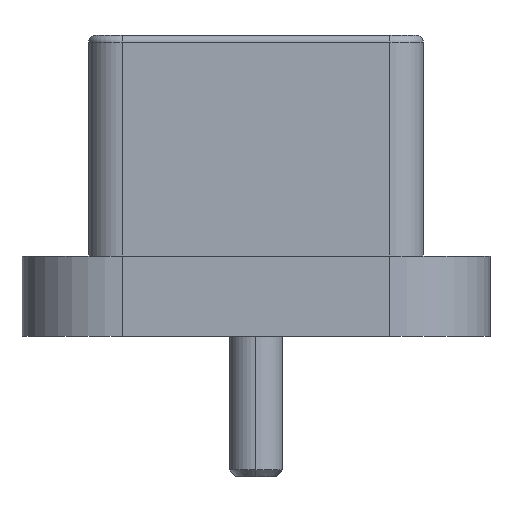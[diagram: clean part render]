
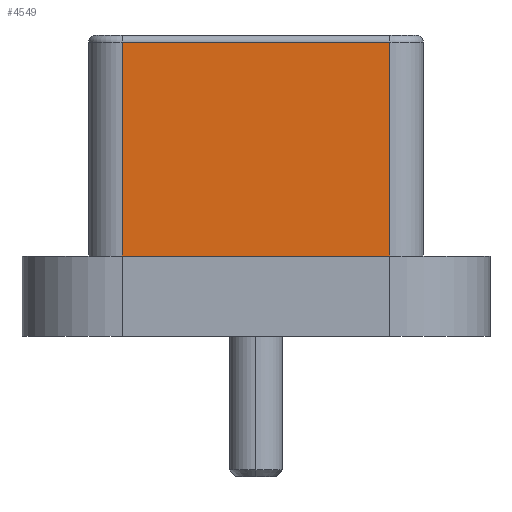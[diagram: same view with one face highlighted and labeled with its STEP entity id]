
A CAD part, left-side view. The second image highlights one B-rep face of the part: STEP entity #4549.
In plain terms, the highlighted planar face has unit normal (-1, 0, 0).
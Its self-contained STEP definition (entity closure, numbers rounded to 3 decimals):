
#329 = DIRECTION ( 'NONE',  ( 0., 1., 0. ) ) ;
#364 = CARTESIAN_POINT ( 'NONE',  ( -9.65, -2., -0.1 ) ) ;
#366 = CARTESIAN_POINT ( 'NONE',  ( -9.65, -2., -3.3 ) ) ;
#398 = LINE ( 'NONE', #364, #2543 ) ;
#404 = AXIS2_PLACEMENT_3D ( 'NONE', #7181, #1972, #4281 ) ;
#947 = VECTOR ( 'NONE', #1927, 1000. ) ;
#1075 = EDGE_CURVE ( 'NONE', #3220, #7100, #398, .T. ) ;
#1433 = EDGE_CURVE ( 'NONE', #1522, #5521, #1969, .T. ) ;
#1522 = VERTEX_POINT ( 'NONE', #6390 ) ;
#1816 = EDGE_CURVE ( 'NONE', #7100, #1522, #2838, .T. ) ;
#1844 = EDGE_CURVE ( 'NONE', #5521, #3220, #6399, .T. ) ;
#1927 = DIRECTION ( 'NONE',  ( 0., -1., 0. ) ) ;
#1964 = CARTESIAN_POINT ( 'NONE',  ( -9.65, 2., -3.3 ) ) ;
#1969 = LINE ( 'NONE', #1964, #947 ) ;
#1972 = DIRECTION ( 'NONE',  ( 1., 0., 0. ) ) ;
#2127 = CARTESIAN_POINT ( 'NONE',  ( -9.65, -2., -0.1 ) ) ;
#2365 = DIRECTION ( 'NONE',  ( 0., 0., -1. ) ) ;
#2540 = FACE_OUTER_BOUND ( 'NONE', #3872, .T. ) ;
#2543 = VECTOR ( 'NONE', #329, 1000. ) ;
#2771 = CARTESIAN_POINT ( 'NONE',  ( -9.65, 2., -0.1 ) ) ;
#2838 = LINE ( 'NONE', #2771, #6101 ) ;
#3220 = VERTEX_POINT ( 'NONE', #2127 ) ;
#3863 = CARTESIAN_POINT ( 'NONE',  ( -9.65, 2., -0.1 ) ) ;
#3872 = EDGE_LOOP ( 'NONE', ( #4864, #4096, #5968, #6753 ) ) ;
#4096 = ORIENTED_EDGE ( 'NONE', *, *, #1433, .T. ) ;
#4281 = DIRECTION ( 'NONE',  ( 0., 1., 0. ) ) ;
#4549 = ADVANCED_FACE ( 'NONE', ( #2540 ), #4852, .F. ) ;
#4852 = PLANE ( 'NONE',  #404 ) ;
#4864 = ORIENTED_EDGE ( 'NONE', *, *, #1816, .T. ) ;
#5521 = VERTEX_POINT ( 'NONE', #366 ) ;
#5968 = ORIENTED_EDGE ( 'NONE', *, *, #1844, .T. ) ;
#6101 = VECTOR ( 'NONE', #2365, 1000. ) ;
#6271 = DIRECTION ( 'NONE',  ( 0., 0., 1. ) ) ;
#6334 = VECTOR ( 'NONE', #6271, 1000. ) ;
#6361 = CARTESIAN_POINT ( 'NONE',  ( -9.65, -2., -3.3 ) ) ;
#6390 = CARTESIAN_POINT ( 'NONE',  ( -9.65, 2., -3.3 ) ) ;
#6399 = LINE ( 'NONE', #6361, #6334 ) ;
#6753 = ORIENTED_EDGE ( 'NONE', *, *, #1075, .T. ) ;
#7100 = VERTEX_POINT ( 'NONE', #3863 ) ;
#7181 = CARTESIAN_POINT ( 'NONE',  ( -9.65, 0., -1.7 ) ) ;
